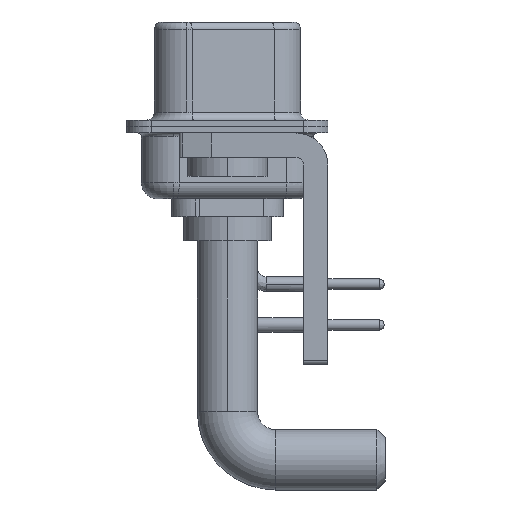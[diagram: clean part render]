
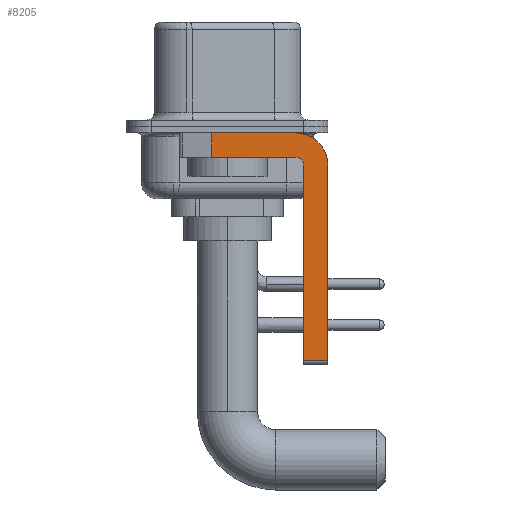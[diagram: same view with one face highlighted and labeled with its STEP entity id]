
A CAD part, left-side view. The second image highlights one B-rep face of the part: STEP entity #8205.
In plain terms, the highlighted planar face has unit normal (-1, 0, 0).
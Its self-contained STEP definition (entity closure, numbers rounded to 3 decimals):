
#35 = EDGE_CURVE ( 'NONE', #1582, #18779, #3939, .T. ) ;
#753 = PLANE ( 'NONE',  #14258 ) ;
#980 = ORIENTED_EDGE ( 'NONE', *, *, #13689, .F. ) ;
#1035 = VERTEX_POINT ( 'NONE', #17283 ) ;
#1499 = ORIENTED_EDGE ( 'NONE', *, *, #7150, .F. ) ;
#1582 = VERTEX_POINT ( 'NONE', #16697 ) ;
#1798 = EDGE_LOOP ( 'NONE', ( #9064, #17269, #980, #5151, #18202, #14948, #1499, #10654 ) ) ;
#1815 = LINE ( 'NONE', #9668, #13789 ) ;
#2014 = CARTESIAN_POINT ( 'NONE',  ( -2.9, 3., -0.4 ) ) ;
#3094 = DIRECTION ( 'NONE',  ( 1., 0., 0. ) ) ;
#3604 = CARTESIAN_POINT ( 'NONE',  ( -2.9, -4.25, -14.55 ) ) ;
#3939 = CIRCLE ( 'NONE', #19551, 2. ) ;
#3993 = CARTESIAN_POINT ( 'NONE',  ( -2.9, -4.25, -2.4 ) ) ;
#4094 = VERTEX_POINT ( 'NONE', #11697 ) ;
#4798 = DIRECTION ( 'NONE',  ( 0., 1., 0. ) ) ;
#4841 = VECTOR ( 'NONE', #18803, 1000. ) ;
#4928 = CARTESIAN_POINT ( 'NONE',  ( -2.9, -4.25, -1.9 ) ) ;
#5151 = ORIENTED_EDGE ( 'NONE', *, *, #7191, .F. ) ;
#5796 = DIRECTION ( 'NONE',  ( 0., 0., -1. ) ) ;
#6882 = CARTESIAN_POINT ( 'NONE',  ( -2.9, -4.25, -1.9 ) ) ;
#7124 = CARTESIAN_POINT ( 'NONE',  ( -2.9, 0.978, -1.9 ) ) ;
#7150 = EDGE_CURVE ( 'NONE', #18779, #8140, #1815, .T. ) ;
#7191 = EDGE_CURVE ( 'NONE', #1035, #15840, #15445, .T. ) ;
#8140 = VERTEX_POINT ( 'NONE', #23923 ) ;
#8205 = ADVANCED_FACE ( 'NONE', ( #9117 ), #753, .F. ) ;
#8374 = CARTESIAN_POINT ( 'NONE',  ( -2.9, -6.25, -2.4 ) ) ;
#9064 = ORIENTED_EDGE ( 'NONE', *, *, #18552, .F. ) ;
#9097 = VERTEX_POINT ( 'NONE', #22651 ) ;
#9117 = FACE_OUTER_BOUND ( 'NONE', #1798, .T. ) ;
#9668 = CARTESIAN_POINT ( 'NONE',  ( -2.9, -6.25, -2.4 ) ) ;
#9872 = DIRECTION ( 'NONE',  ( 0., -1., 0. ) ) ;
#10654 = ORIENTED_EDGE ( 'NONE', *, *, #35, .F. ) ;
#10886 = EDGE_CURVE ( 'NONE', #9097, #8140, #25094, .T. ) ;
#11697 = CARTESIAN_POINT ( 'NONE',  ( -2.9, 0.978, -0.4 ) ) ;
#12445 = VECTOR ( 'NONE', #9872, 1000. ) ;
#12476 = VERTEX_POINT ( 'NONE', #7124 ) ;
#12539 = DIRECTION ( 'NONE',  ( 0., 0., 1. ) ) ;
#12618 = LINE ( 'NONE', #14678, #4841 ) ;
#13243 = DIRECTION ( 'NONE',  ( 0., -1., 0. ) ) ;
#13388 = DIRECTION ( 'NONE',  ( 0., 0., 1. ) ) ;
#13689 = EDGE_CURVE ( 'NONE', #15840, #12476, #18455, .T. ) ;
#13789 = VECTOR ( 'NONE', #5796, 1000. ) ;
#14258 = AXIS2_PLACEMENT_3D ( 'NONE', #14635, #18887, #18375 ) ;
#14359 = CARTESIAN_POINT ( 'NONE',  ( -2.9, -4.75, -14.8 ) ) ;
#14635 = CARTESIAN_POINT ( 'NONE',  ( -2.9, -4.25, -2.4 ) ) ;
#14678 = CARTESIAN_POINT ( 'NONE',  ( -2.9, 0.978, -1.9 ) ) ;
#14948 = ORIENTED_EDGE ( 'NONE', *, *, #10886, .T. ) ;
#15445 = CIRCLE ( 'NONE', #23665, 0.5 ) ;
#15751 = VECTOR ( 'NONE', #12539, 1000. ) ;
#15840 = VERTEX_POINT ( 'NONE', #6882 ) ;
#16477 = DIRECTION ( 'NONE',  ( 0., 0., -1. ) ) ;
#16697 = CARTESIAN_POINT ( 'NONE',  ( -2.9, -4.25, -0.4 ) ) ;
#16857 = CARTESIAN_POINT ( 'NONE',  ( -2.9, -4.25, -2.4 ) ) ;
#17269 = ORIENTED_EDGE ( 'NONE', *, *, #24007, .T. ) ;
#17283 = CARTESIAN_POINT ( 'NONE',  ( -2.9, -4.75, -2.4 ) ) ;
#18202 = ORIENTED_EDGE ( 'NONE', *, *, #18768, .F. ) ;
#18375 = DIRECTION ( 'NONE',  ( 0., 0., -1. ) ) ;
#18455 = LINE ( 'NONE', #4928, #18959 ) ;
#18552 = EDGE_CURVE ( 'NONE', #4094, #1582, #19772, .T. ) ;
#18768 = EDGE_CURVE ( 'NONE', #9097, #1035, #24138, .T. ) ;
#18779 = VERTEX_POINT ( 'NONE', #8374 ) ;
#18803 = DIRECTION ( 'NONE',  ( 0., 0., -1. ) ) ;
#18887 = DIRECTION ( 'NONE',  ( 1., 0., 0. ) ) ;
#18959 = VECTOR ( 'NONE', #4798, 1000. ) ;
#19551 = AXIS2_PLACEMENT_3D ( 'NONE', #16857, #3094, #16477 ) ;
#19772 = LINE ( 'NONE', #2014, #12445 ) ;
#22651 = CARTESIAN_POINT ( 'NONE',  ( -2.9, -4.75, -14.55 ) ) ;
#23417 = VECTOR ( 'NONE', #13243, 1000. ) ;
#23665 = AXIS2_PLACEMENT_3D ( 'NONE', #3993, #25231, #13388 ) ;
#23923 = CARTESIAN_POINT ( 'NONE',  ( -2.9, -6.25, -14.55 ) ) ;
#24007 = EDGE_CURVE ( 'NONE', #4094, #12476, #12618, .T. ) ;
#24138 = LINE ( 'NONE', #14359, #15751 ) ;
#25094 = LINE ( 'NONE', #3604, #23417 ) ;
#25231 = DIRECTION ( 'NONE',  ( -1., 0., 0. ) ) ;
